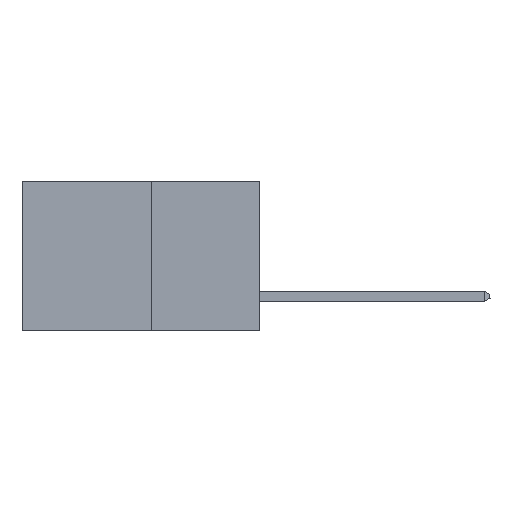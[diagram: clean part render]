
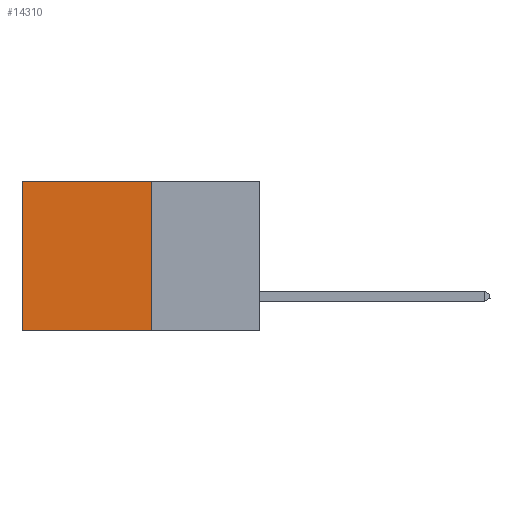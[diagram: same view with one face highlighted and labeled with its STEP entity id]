
A CAD part, left-side view. The second image highlights one B-rep face of the part: STEP entity #14310.
In plain terms, the highlighted planar face has unit normal (-1, 0, 0).
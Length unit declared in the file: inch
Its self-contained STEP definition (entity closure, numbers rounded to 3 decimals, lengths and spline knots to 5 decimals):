
#131 = ORIENTED_EDGE ( 'NONE', *, *, #1713, .T. ) ;
#1102 = AXIS2_PLACEMENT_3D ( 'NONE', #16359, #2491, #12258 ) ;
#1199 = EDGE_LOOP ( 'NONE', ( #131, #4625, #10482, #11021 ) ) ;
#1292 = VECTOR ( 'NONE', #6268, 39.37008 ) ;
#1713 = EDGE_CURVE ( 'NONE', #10125, #6158, #15140, .T. ) ;
#2491 = DIRECTION ( 'NONE',  ( 1., 0., 0. ) ) ;
#2535 = VECTOR ( 'NONE', #14205, 39.37008 ) ;
#3202 = VERTEX_POINT ( 'NONE', #6455 ) ;
#3697 = CARTESIAN_POINT ( 'NONE',  ( 0.277, 0.59, -0.37 ) ) ;
#4625 = ORIENTED_EDGE ( 'NONE', *, *, #11136, .F. ) ;
#4815 = CARTESIAN_POINT ( 'NONE',  ( 0.277, 0.27, 0. ) ) ;
#6102 = DIRECTION ( 'NONE',  ( 0., 0., -1. ) ) ;
#6158 = VERTEX_POINT ( 'NONE', #3697 ) ;
#6268 = DIRECTION ( 'NONE',  ( 0., 1., 0. ) ) ;
#6281 = CARTESIAN_POINT ( 'NONE',  ( 0.277, 0.59, -0.37 ) ) ;
#6455 = CARTESIAN_POINT ( 'NONE',  ( 0.277, 0.27, -0.37 ) ) ;
#6549 = EDGE_CURVE ( 'NONE', #17731, #3202, #13678, .T. ) ;
#6770 = CARTESIAN_POINT ( 'NONE',  ( 0.277, 0.27, 0. ) ) ;
#8835 = LINE ( 'NONE', #4815, #1292 ) ;
#9747 = FACE_OUTER_BOUND ( 'NONE', #1199, .T. ) ;
#10125 = VERTEX_POINT ( 'NONE', #13303 ) ;
#10482 = ORIENTED_EDGE ( 'NONE', *, *, #6549, .F. ) ;
#11021 = ORIENTED_EDGE ( 'NONE', *, *, #17087, .T. ) ;
#11136 = EDGE_CURVE ( 'NONE', #3202, #6158, #17784, .T. ) ;
#12258 = DIRECTION ( 'NONE',  ( 0., 0., -1. ) ) ;
#12427 = DIRECTION ( 'NONE',  ( 0., 1., 0. ) ) ;
#12778 = CARTESIAN_POINT ( 'NONE',  ( 0.277, 0.27, -0.37 ) ) ;
#13303 = CARTESIAN_POINT ( 'NONE',  ( 0.277, 0.59, 0. ) ) ;
#13607 = PLANE ( 'NONE',  #1102 ) ;
#13678 = LINE ( 'NONE', #12778, #2535 ) ;
#14131 = VECTOR ( 'NONE', #12427, 39.37008 ) ;
#14205 = DIRECTION ( 'NONE',  ( 0., 0., -1. ) ) ;
#14310 = ADVANCED_FACE ( 'NONE', ( #9747 ), #13607, .F. ) ;
#15140 = LINE ( 'NONE', #6281, #15573 ) ;
#15573 = VECTOR ( 'NONE', #6102, 39.37008 ) ;
#16359 = CARTESIAN_POINT ( 'NONE',  ( 0.277, 0.27, -0.37 ) ) ;
#16536 = CARTESIAN_POINT ( 'NONE',  ( 0.277, 0.27, -0.37 ) ) ;
#17087 = EDGE_CURVE ( 'NONE', #17731, #10125, #8835, .T. ) ;
#17731 = VERTEX_POINT ( 'NONE', #6770 ) ;
#17784 = LINE ( 'NONE', #16536, #14131 ) ;
